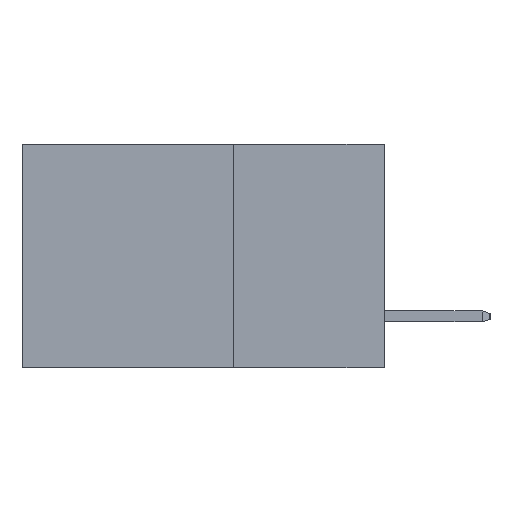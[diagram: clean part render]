
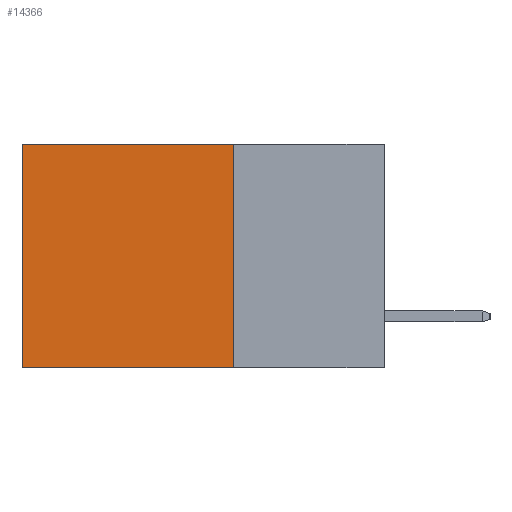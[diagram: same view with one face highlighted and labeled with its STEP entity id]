
A CAD part, left-side view. The second image highlights one B-rep face of the part: STEP entity #14366.
In plain terms, the highlighted planar face has unit normal (-1, 0, 0).
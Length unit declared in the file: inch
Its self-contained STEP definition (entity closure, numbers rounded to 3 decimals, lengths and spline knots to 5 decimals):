
#341 = CARTESIAN_POINT ( 'NONE',  ( 0.2615, 0.25, 0. ) ) ;
#387 = DIRECTION ( 'NONE',  ( 1., 0., 0. ) ) ;
#396 = DIRECTION ( 'NONE',  ( 0., 1., 0. ) ) ;
#958 = AXIS2_PLACEMENT_3D ( 'NONE', #7773, #387, #8971 ) ;
#2428 = EDGE_CURVE ( 'NONE', #2531, #2452, #7457, .T. ) ;
#2452 = VERTEX_POINT ( 'NONE', #9973 ) ;
#2531 = VERTEX_POINT ( 'NONE', #6323 ) ;
#2684 = ORIENTED_EDGE ( 'NONE', *, *, #6972, .T. ) ;
#3731 = EDGE_CURVE ( 'NONE', #12055, #3824, #8377, .T. ) ;
#3824 = VERTEX_POINT ( 'NONE', #7419 ) ;
#4156 = EDGE_CURVE ( 'NONE', #3824, #2452, #8361, .T. ) ;
#6323 = CARTESIAN_POINT ( 'NONE',  ( 0.2615, 0.6, 0. ) ) ;
#6454 = ORIENTED_EDGE ( 'NONE', *, *, #4156, .F. ) ;
#6972 = EDGE_CURVE ( 'NONE', #12055, #2531, #13545, .T. ) ;
#7231 = VECTOR ( 'NONE', #396, 39.37008 ) ;
#7419 = CARTESIAN_POINT ( 'NONE',  ( 0.2615, 0.25, -0.37 ) ) ;
#7457 = LINE ( 'NONE', #13703, #10998 ) ;
#7773 = CARTESIAN_POINT ( 'NONE',  ( 0.2615, 0.25, -0.37 ) ) ;
#7776 = ORIENTED_EDGE ( 'NONE', *, *, #3731, .F. ) ;
#8361 = LINE ( 'NONE', #14556, #14284 ) ;
#8377 = LINE ( 'NONE', #8564, #11161 ) ;
#8477 = DIRECTION ( 'NONE',  ( 0., 0., -1. ) ) ;
#8564 = CARTESIAN_POINT ( 'NONE',  ( 0.2615, 0.25, -0.37 ) ) ;
#8971 = DIRECTION ( 'NONE',  ( 0., 0., -1. ) ) ;
#9610 = DIRECTION ( 'NONE',  ( 0., 0., -1. ) ) ;
#9795 = CARTESIAN_POINT ( 'NONE',  ( 0.2615, 0.25, 0. ) ) ;
#9973 = CARTESIAN_POINT ( 'NONE',  ( 0.2615, 0.6, -0.37 ) ) ;
#10998 = VECTOR ( 'NONE', #9610, 39.37008 ) ;
#11161 = VECTOR ( 'NONE', #8477, 39.37008 ) ;
#11375 = FACE_OUTER_BOUND ( 'NONE', #13986, .T. ) ;
#12055 = VERTEX_POINT ( 'NONE', #9795 ) ;
#12463 = ORIENTED_EDGE ( 'NONE', *, *, #2428, .T. ) ;
#13545 = LINE ( 'NONE', #341, #7231 ) ;
#13680 = PLANE ( 'NONE',  #958 ) ;
#13703 = CARTESIAN_POINT ( 'NONE',  ( 0.2615, 0.6, -0.37 ) ) ;
#13986 = EDGE_LOOP ( 'NONE', ( #12463, #6454, #7776, #2684 ) ) ;
#14284 = VECTOR ( 'NONE', #14574, 39.37008 ) ;
#14366 = ADVANCED_FACE ( 'NONE', ( #11375 ), #13680, .F. ) ;
#14556 = CARTESIAN_POINT ( 'NONE',  ( 0.2615, 0.25, -0.37 ) ) ;
#14574 = DIRECTION ( 'NONE',  ( 0., 1., 0. ) ) ;
